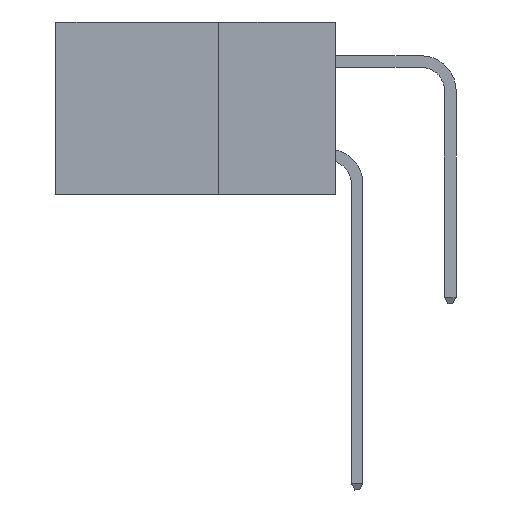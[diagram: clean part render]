
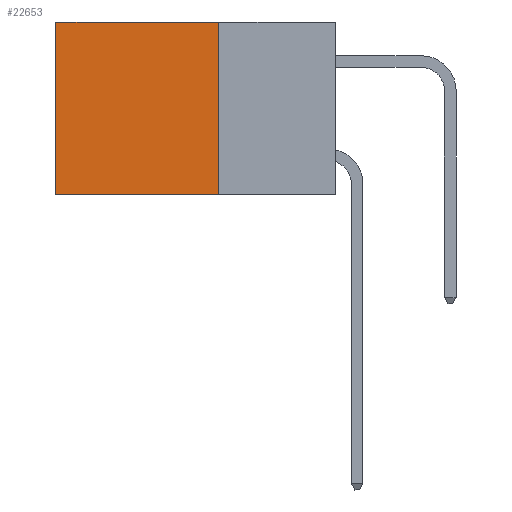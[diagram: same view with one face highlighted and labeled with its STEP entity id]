
A CAD part, left-side view. The second image highlights one B-rep face of the part: STEP entity #22653.
In plain terms, the highlighted planar face has unit normal (-1, 0, 0).
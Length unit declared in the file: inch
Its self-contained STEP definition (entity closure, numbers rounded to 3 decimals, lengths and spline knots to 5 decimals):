
#391 = FACE_OUTER_BOUND ( 'NONE', #30255, .T. ) ;
#772 = VECTOR ( 'NONE', #8842, 39.37008 ) ;
#4156 = LINE ( 'NONE', #34032, #772 ) ;
#7846 = ORIENTED_EDGE ( 'NONE', *, *, #15647, .F. ) ;
#8842 = DIRECTION ( 'NONE',  ( 0., 0., -1. ) ) ;
#8940 = CARTESIAN_POINT ( 'NONE',  ( 0.2875, 0.6, -0.37 ) ) ;
#9571 = VERTEX_POINT ( 'NONE', #12701 ) ;
#10331 = DIRECTION ( 'NONE',  ( 0., 1., 0. ) ) ;
#11179 = VERTEX_POINT ( 'NONE', #8940 ) ;
#12697 = VECTOR ( 'NONE', #35472, 39.37008 ) ;
#12701 = CARTESIAN_POINT ( 'NONE',  ( 0.2875, 0.6, 0. ) ) ;
#12728 = VECTOR ( 'NONE', #10331, 39.37008 ) ;
#12843 = VECTOR ( 'NONE', #33405, 39.37008 ) ;
#13251 = CARTESIAN_POINT ( 'NONE',  ( 0.2875, 0.25, 0. ) ) ;
#13384 = EDGE_CURVE ( 'NONE', #26362, #13754, #4156, .T. ) ;
#13754 = VERTEX_POINT ( 'NONE', #16615 ) ;
#14402 = EDGE_CURVE ( 'NONE', #9571, #11179, #23133, .T. ) ;
#15647 = EDGE_CURVE ( 'NONE', #13754, #11179, #28947, .T. ) ;
#16105 = LINE ( 'NONE', #32729, #12697 ) ;
#16615 = CARTESIAN_POINT ( 'NONE',  ( 0.2875, 0.25, -0.37 ) ) ;
#17077 = ORIENTED_EDGE ( 'NONE', *, *, #13384, .F. ) ;
#18254 = AXIS2_PLACEMENT_3D ( 'NONE', #19549, #35197, #22449 ) ;
#18489 = PLANE ( 'NONE',  #18254 ) ;
#19549 = CARTESIAN_POINT ( 'NONE',  ( 0.2875, 0.25, 0. ) ) ;
#21284 = EDGE_CURVE ( 'NONE', #26362, #9571, #16105, .T. ) ;
#22449 = DIRECTION ( 'NONE',  ( 0., 0., -1. ) ) ;
#22653 = ADVANCED_FACE ( 'NONE', ( #391 ), #18489, .F. ) ;
#23133 = LINE ( 'NONE', #36030, #12843 ) ;
#26362 = VERTEX_POINT ( 'NONE', #13251 ) ;
#28947 = LINE ( 'NONE', #38786, #12728 ) ;
#30255 = EDGE_LOOP ( 'NONE', ( #37925, #7846, #17077, #33477 ) ) ;
#32729 = CARTESIAN_POINT ( 'NONE',  ( 0.2875, 0.25, 0. ) ) ;
#33405 = DIRECTION ( 'NONE',  ( 0., 0., -1. ) ) ;
#33477 = ORIENTED_EDGE ( 'NONE', *, *, #21284, .T. ) ;
#34032 = CARTESIAN_POINT ( 'NONE',  ( 0.2875, 0.25, 0. ) ) ;
#35197 = DIRECTION ( 'NONE',  ( 1., 0., 0. ) ) ;
#35472 = DIRECTION ( 'NONE',  ( 0., 1., 0. ) ) ;
#36030 = CARTESIAN_POINT ( 'NONE',  ( 0.2875, 0.6, 0. ) ) ;
#37925 = ORIENTED_EDGE ( 'NONE', *, *, #14402, .T. ) ;
#38786 = CARTESIAN_POINT ( 'NONE',  ( 0.2875, 0.25, -0.37 ) ) ;
